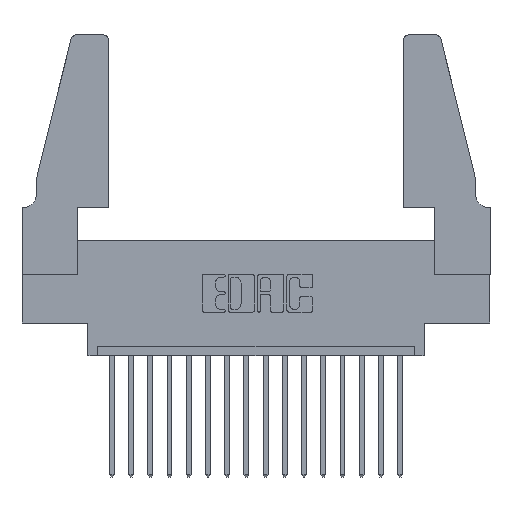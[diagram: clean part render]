
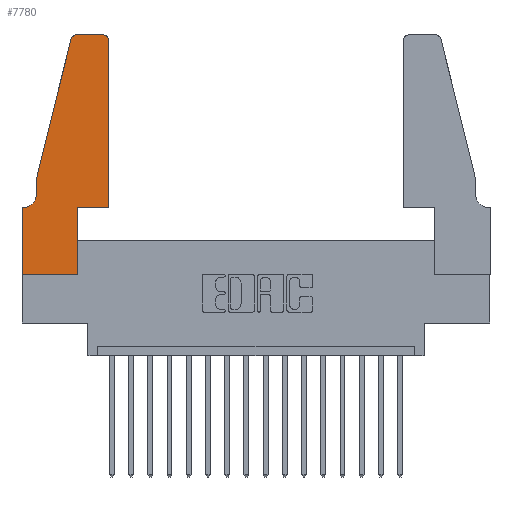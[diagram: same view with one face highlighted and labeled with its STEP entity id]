
A CAD part, top view. The second image highlights one B-rep face of the part: STEP entity #7780.
In plain terms, the highlighted planar face has unit normal (0, 0, 1).
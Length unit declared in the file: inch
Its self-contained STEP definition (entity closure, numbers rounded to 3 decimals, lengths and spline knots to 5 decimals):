
#114 = ORIENTED_EDGE ( 'NONE', *, *, #6597, .T. ) ;
#309 = CARTESIAN_POINT ( 'NONE',  ( 0.4205, 1.22, 0.37 ) ) ;
#371 = DIRECTION ( 'NONE',  ( 1., 0., 0. ) ) ;
#378 = ORIENTED_EDGE ( 'NONE', *, *, #15250, .T. ) ;
#499 = DIRECTION ( 'NONE',  ( -1., 0., 0. ) ) ;
#755 = LINE ( 'NONE', #6350, #14949 ) ;
#1315 = DIRECTION ( 'NONE',  ( 0., -1., 0. ) ) ;
#1319 = CARTESIAN_POINT ( 'NONE',  ( 0., 0., 0.37 ) ) ;
#1457 = CARTESIAN_POINT ( 'NONE',  ( 0.4505, 0.35, 0.37 ) ) ;
#1681 = ORIENTED_EDGE ( 'NONE', *, *, #5637, .T. ) ;
#1732 = VECTOR ( 'NONE', #14856, 39.37008 ) ;
#1991 = LINE ( 'NONE', #8572, #16210 ) ;
#2225 = CARTESIAN_POINT ( 'NONE',  ( 0.0055, 0.35, 0.37 ) ) ;
#2925 = EDGE_CURVE ( 'NONE', #9282, #6259, #755, .T. ) ;
#3126 = DIRECTION ( 'NONE',  ( -1., 0., 0. ) ) ;
#3436 = AXIS2_PLACEMENT_3D ( 'NONE', #309, #8615, #371 ) ;
#3861 = DIRECTION ( 'NONE',  ( 0., 0., 1. ) ) ;
#3966 = CARTESIAN_POINT ( 'NONE',  ( 0.2865, 0., 0.37 ) ) ;
#4023 = VERTEX_POINT ( 'NONE', #11339 ) ;
#4248 = EDGE_LOOP ( 'NONE', ( #9344, #1681, #14020, #378, #9005, #7434, #13374, #14539, #13845, #10556, #114, #7023 ) ) ;
#4442 = CARTESIAN_POINT ( 'NONE',  ( 0., 0.35, 0.37 ) ) ;
#4709 = CARTESIAN_POINT ( 'NONE',  ( 0.0755, 0.42, 0.37 ) ) ;
#4739 = LINE ( 'NONE', #6738, #15255 ) ;
#4765 = VERTEX_POINT ( 'NONE', #2225 ) ;
#4938 = EDGE_CURVE ( 'NONE', #11243, #15024, #6296, .T. ) ;
#4985 = DIRECTION ( 'NONE',  ( 0., 1., 0. ) ) ;
#5637 = EDGE_CURVE ( 'NONE', #6259, #11243, #16326, .T. ) ;
#6021 = CIRCLE ( 'NONE', #3436, 0.03 ) ;
#6163 = VECTOR ( 'NONE', #4985, 39.37008 ) ;
#6259 = VERTEX_POINT ( 'NONE', #13473 ) ;
#6296 = LINE ( 'NONE', #15256, #14888 ) ;
#6350 = CARTESIAN_POINT ( 'NONE',  ( 0.2605, 1.25, 0.37 ) ) ;
#6367 = CARTESIAN_POINT ( 'NONE',  ( 0.0755, 0.5, 0.37 ) ) ;
#6597 = EDGE_CURVE ( 'NONE', #9883, #4023, #10021, .T. ) ;
#6738 = CARTESIAN_POINT ( 'NONE',  ( 0., 0., 0.37 ) ) ;
#6932 = CARTESIAN_POINT ( 'NONE',  ( 0.284, 1.22, 0.37 ) ) ;
#7023 = ORIENTED_EDGE ( 'NONE', *, *, #9881, .T. ) ;
#7434 = ORIENTED_EDGE ( 'NONE', *, *, #8344, .T. ) ;
#7780 = ADVANCED_FACE ( 'NONE', ( #12322 ), #10152, .T. ) ;
#8075 = EDGE_CURVE ( 'NONE', #15444, #17704, #10402, .T. ) ;
#8344 = EDGE_CURVE ( 'NONE', #4765, #8379, #1991, .T. ) ;
#8379 = VERTEX_POINT ( 'NONE', #4442 ) ;
#8411 = EDGE_CURVE ( 'NONE', #11704, #9883, #9096, .T. ) ;
#8454 = CIRCLE ( 'NONE', #9534, 0.07 ) ;
#8572 = CARTESIAN_POINT ( 'NONE',  ( 0.0755, 0.35, 0.37 ) ) ;
#8574 = DIRECTION ( 'NONE',  ( 0., -1., 0. ) ) ;
#8615 = DIRECTION ( 'NONE',  ( 0., 0., 1. ) ) ;
#9005 = ORIENTED_EDGE ( 'NONE', *, *, #15865, .T. ) ;
#9096 = LINE ( 'NONE', #16163, #15973 ) ;
#9282 = VERTEX_POINT ( 'NONE', #16304 ) ;
#9302 = CARTESIAN_POINT ( 'NONE',  ( 0.4505, 0.35, 0.37 ) ) ;
#9337 = EDGE_CURVE ( 'NONE', #17704, #11704, #13792, .T. ) ;
#9344 = ORIENTED_EDGE ( 'NONE', *, *, #2925, .T. ) ;
#9422 = DIRECTION ( 'NONE',  ( 1., 0., 0. ) ) ;
#9534 = AXIS2_PLACEMENT_3D ( 'NONE', #12993, #16996, #499 ) ;
#9576 = AXIS2_PLACEMENT_3D ( 'NONE', #6932, #12330, #9422 ) ;
#9881 = EDGE_CURVE ( 'NONE', #4023, #9282, #6021, .T. ) ;
#9883 = VERTEX_POINT ( 'NONE', #1457 ) ;
#9927 = CARTESIAN_POINT ( 'NONE',  ( 0.25487, 1.22718, 0.37 ) ) ;
#10021 = LINE ( 'NONE', #9302, #6163 ) ;
#10139 = CARTESIAN_POINT ( 'NONE',  ( 0.0755, 0.5, 0.37 ) ) ;
#10152 = PLANE ( 'NONE',  #12430 ) ;
#10402 = LINE ( 'NONE', #12178, #14919 ) ;
#10556 = ORIENTED_EDGE ( 'NONE', *, *, #8411, .T. ) ;
#10723 = EDGE_CURVE ( 'NONE', #8379, #15444, #4739, .T. ) ;
#11243 = VERTEX_POINT ( 'NONE', #9927 ) ;
#11339 = CARTESIAN_POINT ( 'NONE',  ( 0.4505, 1.22, 0.37 ) ) ;
#11704 = VERTEX_POINT ( 'NONE', #13944 ) ;
#12123 = DIRECTION ( 'NONE',  ( 1., 0., 0. ) ) ;
#12178 = CARTESIAN_POINT ( 'NONE',  ( 0., 0., 0.37 ) ) ;
#12322 = FACE_OUTER_BOUND ( 'NONE', #4248, .T. ) ;
#12330 = DIRECTION ( 'NONE',  ( 0., 0., 1. ) ) ;
#12359 = DIRECTION ( 'NONE',  ( -0.239, -0.971, 0. ) ) ;
#12430 = AXIS2_PLACEMENT_3D ( 'NONE', #14306, #3861, #13212 ) ;
#12993 = CARTESIAN_POINT ( 'NONE',  ( 0.0055, 0.42, 0.37 ) ) ;
#13186 = DIRECTION ( 'NONE',  ( -1., 0., 0. ) ) ;
#13212 = DIRECTION ( 'NONE',  ( 1., 0., 0. ) ) ;
#13374 = ORIENTED_EDGE ( 'NONE', *, *, #10723, .T. ) ;
#13444 = DIRECTION ( 'NONE',  ( 1., 0., 0. ) ) ;
#13473 = CARTESIAN_POINT ( 'NONE',  ( 0.284, 1.25, 0.37 ) ) ;
#13792 = LINE ( 'NONE', #17707, #1732 ) ;
#13845 = ORIENTED_EDGE ( 'NONE', *, *, #9337, .T. ) ;
#13944 = CARTESIAN_POINT ( 'NONE',  ( 0.2865, 0.35, 0.37 ) ) ;
#14020 = ORIENTED_EDGE ( 'NONE', *, *, #4938, .T. ) ;
#14306 = CARTESIAN_POINT ( 'NONE',  ( 0., 0.35, 0.37 ) ) ;
#14539 = ORIENTED_EDGE ( 'NONE', *, *, #8075, .T. ) ;
#14856 = DIRECTION ( 'NONE',  ( 0., 1., 0. ) ) ;
#14888 = VECTOR ( 'NONE', #12359, 39.37008 ) ;
#14919 = VECTOR ( 'NONE', #12123, 39.37008 ) ;
#14949 = VECTOR ( 'NONE', #13186, 39.37008 ) ;
#15024 = VERTEX_POINT ( 'NONE', #6367 ) ;
#15141 = LINE ( 'NONE', #10139, #17778 ) ;
#15250 = EDGE_CURVE ( 'NONE', #15024, #16657, #15141, .T. ) ;
#15255 = VECTOR ( 'NONE', #1315, 39.37008 ) ;
#15256 = CARTESIAN_POINT ( 'NONE',  ( 0.0755, 0.5, 0.37 ) ) ;
#15444 = VERTEX_POINT ( 'NONE', #1319 ) ;
#15865 = EDGE_CURVE ( 'NONE', #16657, #4765, #8454, .T. ) ;
#15973 = VECTOR ( 'NONE', #13444, 39.37008 ) ;
#16163 = CARTESIAN_POINT ( 'NONE',  ( 0.4505, 0.35, 0.37 ) ) ;
#16210 = VECTOR ( 'NONE', #3126, 39.37008 ) ;
#16304 = CARTESIAN_POINT ( 'NONE',  ( 0.4205, 1.25, 0.37 ) ) ;
#16326 = CIRCLE ( 'NONE', #9576, 0.03 ) ;
#16657 = VERTEX_POINT ( 'NONE', #4709 ) ;
#16996 = DIRECTION ( 'NONE',  ( 0., 0., -1. ) ) ;
#17704 = VERTEX_POINT ( 'NONE', #3966 ) ;
#17707 = CARTESIAN_POINT ( 'NONE',  ( 0.2865, 0.35, 0.37 ) ) ;
#17778 = VECTOR ( 'NONE', #8574, 39.37008 ) ;
